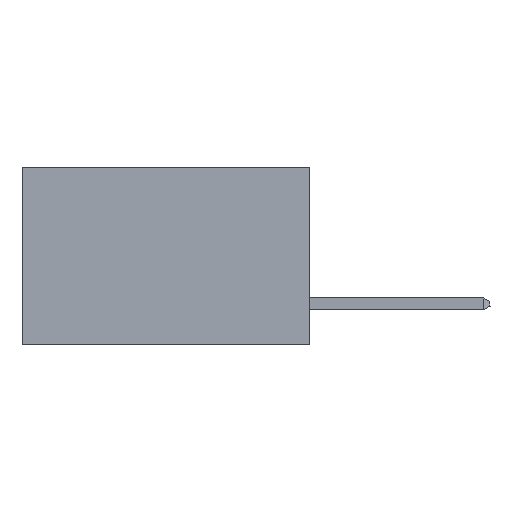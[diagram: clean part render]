
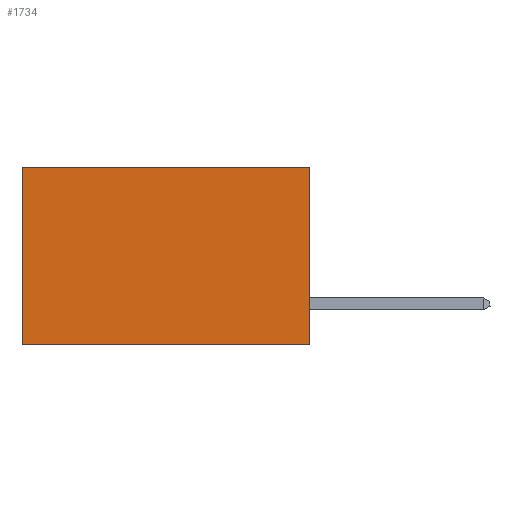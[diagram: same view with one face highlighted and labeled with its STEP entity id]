
A CAD part, left-side view. The second image highlights one B-rep face of the part: STEP entity #1734.
In plain terms, the highlighted planar face has unit normal (-1, 0, 0).
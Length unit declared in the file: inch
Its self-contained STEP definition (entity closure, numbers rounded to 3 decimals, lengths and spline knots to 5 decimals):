
#274 = ORIENTED_EDGE ( 'NONE', *, *, #9121, .T. ) ;
#435 = CARTESIAN_POINT ( 'NONE',  ( 0.2875, 0., -0.37 ) ) ;
#892 = CARTESIAN_POINT ( 'NONE',  ( 0.2875, 0.6, 0. ) ) ;
#1051 = PLANE ( 'NONE',  #9373 ) ;
#1734 = ADVANCED_FACE ( 'NONE', ( #16768 ), #1051, .F. ) ;
#3097 = CARTESIAN_POINT ( 'NONE',  ( 0.2875, 0., -0.37 ) ) ;
#3111 = CARTESIAN_POINT ( 'NONE',  ( 0.2875, 0.6, -0.37 ) ) ;
#3755 = CARTESIAN_POINT ( 'NONE',  ( 0.2875, 0., 0. ) ) ;
#4419 = EDGE_LOOP ( 'NONE', ( #274, #13130, #8802, #15911 ) ) ;
#4701 = VERTEX_POINT ( 'NONE', #3111 ) ;
#5044 = VERTEX_POINT ( 'NONE', #435 ) ;
#5251 = VECTOR ( 'NONE', #16791, 39.37008 ) ;
#7301 = DIRECTION ( 'NONE',  ( 0., 1., 0. ) ) ;
#8149 = CARTESIAN_POINT ( 'NONE',  ( 0.2875, 0., 0. ) ) ;
#8219 = DIRECTION ( 'NONE',  ( 0., 1., 0. ) ) ;
#8802 = ORIENTED_EDGE ( 'NONE', *, *, #10188, .F. ) ;
#9121 = EDGE_CURVE ( 'NONE', #17155, #4701, #15620, .T. ) ;
#9201 = VERTEX_POINT ( 'NONE', #3755 ) ;
#9373 = AXIS2_PLACEMENT_3D ( 'NONE', #8149, #12734, #15724 ) ;
#10188 = EDGE_CURVE ( 'NONE', #9201, #5044, #12781, .T. ) ;
#10920 = CARTESIAN_POINT ( 'NONE',  ( 0.2875, 0., 0. ) ) ;
#12180 = LINE ( 'NONE', #12603, #14049 ) ;
#12218 = EDGE_CURVE ( 'NONE', #5044, #4701, #13423, .T. ) ;
#12603 = CARTESIAN_POINT ( 'NONE',  ( 0.2875, 0., 0. ) ) ;
#12734 = DIRECTION ( 'NONE',  ( 1., 0., 0. ) ) ;
#12781 = LINE ( 'NONE', #10920, #13484 ) ;
#13130 = ORIENTED_EDGE ( 'NONE', *, *, #12218, .F. ) ;
#13423 = LINE ( 'NONE', #3097, #16190 ) ;
#13484 = VECTOR ( 'NONE', #15926, 39.37008 ) ;
#13574 = EDGE_CURVE ( 'NONE', #9201, #17155, #12180, .T. ) ;
#13581 = CARTESIAN_POINT ( 'NONE',  ( 0.2875, 0.6, 0. ) ) ;
#14049 = VECTOR ( 'NONE', #8219, 39.37008 ) ;
#15620 = LINE ( 'NONE', #892, #5251 ) ;
#15724 = DIRECTION ( 'NONE',  ( 0., 0., -1. ) ) ;
#15911 = ORIENTED_EDGE ( 'NONE', *, *, #13574, .T. ) ;
#15926 = DIRECTION ( 'NONE',  ( 0., 0., -1. ) ) ;
#16190 = VECTOR ( 'NONE', #7301, 39.37008 ) ;
#16768 = FACE_OUTER_BOUND ( 'NONE', #4419, .T. ) ;
#16791 = DIRECTION ( 'NONE',  ( 0., 0., -1. ) ) ;
#17155 = VERTEX_POINT ( 'NONE', #13581 ) ;
